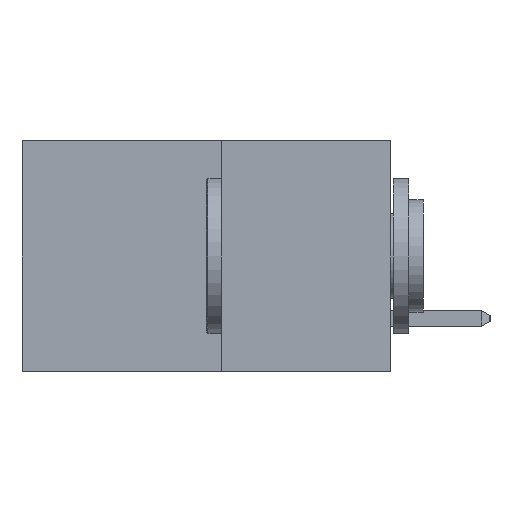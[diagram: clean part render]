
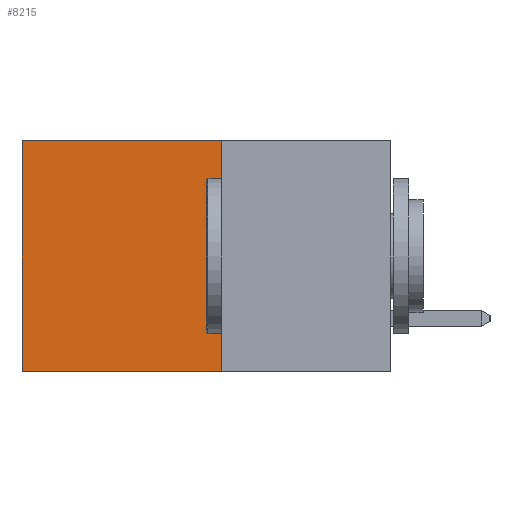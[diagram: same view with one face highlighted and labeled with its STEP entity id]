
A CAD part, left-side view. The second image highlights one B-rep face of the part: STEP entity #8215.
In plain terms, the highlighted planar face has unit normal (-1, 0, 0).
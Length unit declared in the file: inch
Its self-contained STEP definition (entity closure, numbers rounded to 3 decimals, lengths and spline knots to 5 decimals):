
#484 = CARTESIAN_POINT ( 'NONE',  ( 0.277, 0.27, 0. ) ) ;
#745 = CARTESIAN_POINT ( 'NONE',  ( 0.277, 0.59, -0.37 ) ) ;
#2320 = CARTESIAN_POINT ( 'NONE',  ( 0.277, 0.59, -0.37 ) ) ;
#2577 = LINE ( 'NONE', #484, #11748 ) ;
#2933 = CARTESIAN_POINT ( 'NONE',  ( 0.277, 0.27, 0. ) ) ;
#3545 = LINE ( 'NONE', #13726, #24811 ) ;
#4561 = VERTEX_POINT ( 'NONE', #2320 ) ;
#5348 = LINE ( 'NONE', #24609, #15077 ) ;
#6375 = AXIS2_PLACEMENT_3D ( 'NONE', #21593, #23597, #11369 ) ;
#6853 = DIRECTION ( 'NONE',  ( 0., 1., 0. ) ) ;
#8215 = ADVANCED_FACE ( 'NONE', ( #12383 ), #9297, .F. ) ;
#9297 = PLANE ( 'NONE',  #6375 ) ;
#10403 = EDGE_CURVE ( 'NONE', #12199, #4561, #16379, .T. ) ;
#11369 = DIRECTION ( 'NONE',  ( 0., 0., -1. ) ) ;
#11748 = VECTOR ( 'NONE', #6853, 39.37008 ) ;
#12199 = VERTEX_POINT ( 'NONE', #15818 ) ;
#12383 = FACE_OUTER_BOUND ( 'NONE', #23651, .T. ) ;
#12634 = EDGE_CURVE ( 'NONE', #22598, #12199, #2577, .T. ) ;
#13364 = VERTEX_POINT ( 'NONE', #21311 ) ;
#13726 = CARTESIAN_POINT ( 'NONE',  ( 0.277, 0.27, -0.37 ) ) ;
#15077 = VECTOR ( 'NONE', #16438, 39.37008 ) ;
#15340 = DIRECTION ( 'NONE',  ( 0., 0., -1. ) ) ;
#15791 = DIRECTION ( 'NONE',  ( 0., 1., 0. ) ) ;
#15818 = CARTESIAN_POINT ( 'NONE',  ( 0.277, 0.59, 0. ) ) ;
#16379 = LINE ( 'NONE', #745, #22433 ) ;
#16438 = DIRECTION ( 'NONE',  ( 0., 0., -1. ) ) ;
#16793 = EDGE_CURVE ( 'NONE', #22598, #13364, #5348, .T. ) ;
#19818 = ORIENTED_EDGE ( 'NONE', *, *, #16793, .F. ) ;
#21311 = CARTESIAN_POINT ( 'NONE',  ( 0.277, 0.27, -0.37 ) ) ;
#21403 = ORIENTED_EDGE ( 'NONE', *, *, #12634, .T. ) ;
#21593 = CARTESIAN_POINT ( 'NONE',  ( 0.277, 0.27, -0.37 ) ) ;
#22433 = VECTOR ( 'NONE', #15340, 39.37008 ) ;
#22598 = VERTEX_POINT ( 'NONE', #2933 ) ;
#23343 = ORIENTED_EDGE ( 'NONE', *, *, #24621, .F. ) ;
#23597 = DIRECTION ( 'NONE',  ( 1., 0., 0. ) ) ;
#23651 = EDGE_LOOP ( 'NONE', ( #25353, #23343, #19818, #21403 ) ) ;
#24609 = CARTESIAN_POINT ( 'NONE',  ( 0.277, 0.27, -0.37 ) ) ;
#24621 = EDGE_CURVE ( 'NONE', #13364, #4561, #3545, .T. ) ;
#24811 = VECTOR ( 'NONE', #15791, 39.37008 ) ;
#25353 = ORIENTED_EDGE ( 'NONE', *, *, #10403, .T. ) ;
